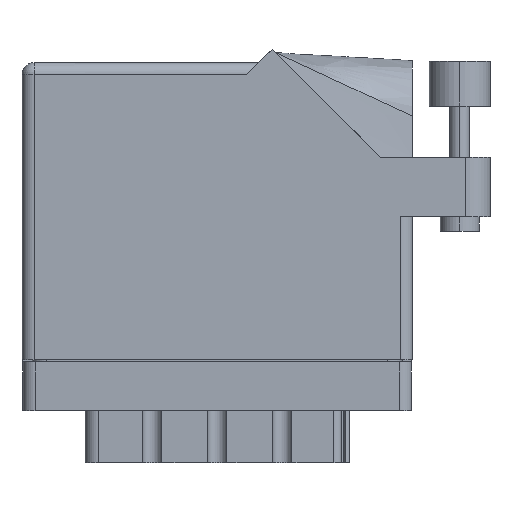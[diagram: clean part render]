
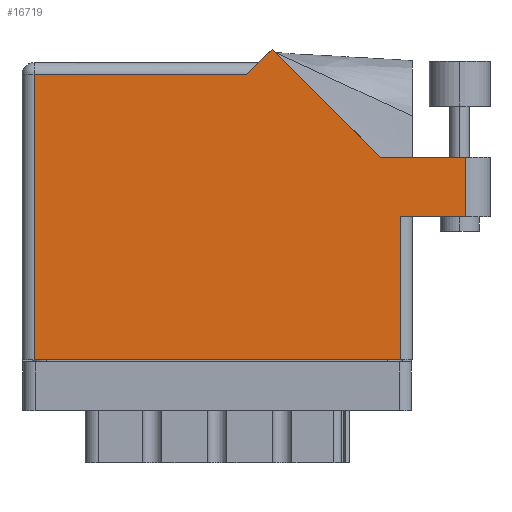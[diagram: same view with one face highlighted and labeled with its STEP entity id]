
A CAD part, front view. The second image highlights one B-rep face of the part: STEP entity #16719.
In plain terms, the highlighted face is planar.
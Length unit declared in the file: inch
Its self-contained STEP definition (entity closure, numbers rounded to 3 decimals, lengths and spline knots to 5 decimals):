
#139 = VERTEX_POINT ( 'NONE', #1897 ) ;
#693 = EDGE_CURVE ( 'NONE', #36157, #2123, #4992, .T. ) ;
#809 = CARTESIAN_POINT ( 'NONE',  ( 2.285, 1.044, 0. ) ) ;
#1897 = CARTESIAN_POINT ( 'NONE',  ( 1.948, 0., 0. ) ) ;
#2123 = VERTEX_POINT ( 'NONE', #23242 ) ;
#2434 = CARTESIAN_POINT ( 'NONE',  ( 1.155, 1.468, 0. ) ) ;
#3070 = VERTEX_POINT ( 'NONE', #40826 ) ;
#3728 = VERTEX_POINT ( 'NONE', #4222 ) ;
#4073 = VECTOR ( 'NONE', #17638, 39.37008 ) ;
#4222 = CARTESIAN_POINT ( 'NONE',  ( 0.062, 1.468, 0. ) ) ;
#4380 = CARTESIAN_POINT ( 'NONE',  ( 1.948, 0.737, 0. ) ) ;
#4992 = LINE ( 'NONE', #37120, #35378 ) ;
#5123 = VECTOR ( 'NONE', #17401, 39.37008 ) ;
#5252 = VERTEX_POINT ( 'NONE', #12595 ) ;
#5459 = EDGE_CURVE ( 'NONE', #139, #3070, #6660, .T. ) ;
#5875 = VERTEX_POINT ( 'NONE', #35113 ) ;
#5968 = DIRECTION ( 'NONE',  ( -1., 0., 0. ) ) ;
#6402 = DIRECTION ( 'NONE',  ( -1., 0., 0. ) ) ;
#6660 = LINE ( 'NONE', #4380, #40478 ) ;
#6796 = DIRECTION ( 'NONE',  ( 0., -1., 0. ) ) ;
#6895 = EDGE_CURVE ( 'NONE', #3070, #5252, #36879, .T. ) ;
#7743 = CARTESIAN_POINT ( 'NONE',  ( 2.01, 0.737, 0. ) ) ;
#8780 = LINE ( 'NONE', #33795, #28746 ) ;
#10447 = VECTOR ( 'NONE', #6796, 39.37008 ) ;
#10452 = CARTESIAN_POINT ( 'NONE',  ( 1.84442, 1.044, 0. ) ) ;
#10543 = EDGE_CURVE ( 'NONE', #2123, #13192, #39895, .T. ) ;
#10945 = DIRECTION ( 'NONE',  ( 1., 0., 0. ) ) ;
#11374 = CARTESIAN_POINT ( 'NONE',  ( 2.285, 1.044, 0. ) ) ;
#12034 = EDGE_CURVE ( 'NONE', #20595, #36157, #25389, .T. ) ;
#12595 = CARTESIAN_POINT ( 'NONE',  ( 2.285, 0.737, 0. ) ) ;
#13192 = VERTEX_POINT ( 'NONE', #2434 ) ;
#13407 = EDGE_LOOP ( 'NONE', ( #14334, #23855, #37479, #35496, #15533, #14873, #13484, #30137, #29084 ) ) ;
#13484 = ORIENTED_EDGE ( 'NONE', *, *, #17842, .T. ) ;
#13497 = VECTOR ( 'NONE', #10945, 39.37008 ) ;
#14334 = ORIENTED_EDGE ( 'NONE', *, *, #6895, .T. ) ;
#14409 = CARTESIAN_POINT ( 'NONE',  ( 1.217, 1.53, 0. ) ) ;
#14873 = ORIENTED_EDGE ( 'NONE', *, *, #29199, .T. ) ;
#15533 = ORIENTED_EDGE ( 'NONE', *, *, #10543, .T. ) ;
#15965 = LINE ( 'NONE', #25849, #10447 ) ;
#16445 = VECTOR ( 'NONE', #6402, 39.37008 ) ;
#16719 = ADVANCED_FACE ( 'NONE', ( #32249 ), #24894, .F. ) ;
#17401 = DIRECTION ( 'NONE',  ( 0., 1., 0. ) ) ;
#17638 = DIRECTION ( 'NONE',  ( -0.707, -0.707, 0. ) ) ;
#17842 = EDGE_CURVE ( 'NONE', #3728, #5875, #15965, .T. ) ;
#20595 = VERTEX_POINT ( 'NONE', #11374 ) ;
#23242 = CARTESIAN_POINT ( 'NONE',  ( 1.28771, 1.60071, 0. ) ) ;
#23855 = ORIENTED_EDGE ( 'NONE', *, *, #27648, .T. ) ;
#24351 = DIRECTION ( 'NONE',  ( -0.707, 0.707, 0. ) ) ;
#24894 = PLANE ( 'NONE',  #34003 ) ;
#25389 = LINE ( 'NONE', #25464, #16445 ) ;
#25464 = CARTESIAN_POINT ( 'NONE',  ( 2.41, 1.044, 0. ) ) ;
#25849 = CARTESIAN_POINT ( 'NONE',  ( 0.062, 0., 0. ) ) ;
#26364 = VECTOR ( 'NONE', #31469, 39.37008 ) ;
#27648 = EDGE_CURVE ( 'NONE', #5252, #20595, #32977, .T. ) ;
#28746 = VECTOR ( 'NONE', #37788, 39.37008 ) ;
#29084 = ORIENTED_EDGE ( 'NONE', *, *, #5459, .T. ) ;
#29199 = EDGE_CURVE ( 'NONE', #13192, #3728, #35820, .T. ) ;
#30137 = ORIENTED_EDGE ( 'NONE', *, *, #31754, .T. ) ;
#31206 = CARTESIAN_POINT ( 'NONE',  ( 0., 1.468, 0. ) ) ;
#31469 = DIRECTION ( 'NONE',  ( -1., 0., 0. ) ) ;
#31754 = EDGE_CURVE ( 'NONE', #5875, #139, #8780, .T. ) ;
#32249 = FACE_OUTER_BOUND ( 'NONE', #13407, .T. ) ;
#32775 = DIRECTION ( 'NONE',  ( 0., 1., 0. ) ) ;
#32977 = LINE ( 'NONE', #809, #5123 ) ;
#33795 = CARTESIAN_POINT ( 'NONE',  ( 0., 0., 0. ) ) ;
#34003 = AXIS2_PLACEMENT_3D ( 'NONE', #37796, #38223, #5968 ) ;
#35113 = CARTESIAN_POINT ( 'NONE',  ( 0.062, 0., 0. ) ) ;
#35378 = VECTOR ( 'NONE', #24351, 39.37008 ) ;
#35496 = ORIENTED_EDGE ( 'NONE', *, *, #693, .T. ) ;
#35820 = LINE ( 'NONE', #31206, #26364 ) ;
#36157 = VERTEX_POINT ( 'NONE', #10452 ) ;
#36879 = LINE ( 'NONE', #7743, #13497 ) ;
#37120 = CARTESIAN_POINT ( 'NONE',  ( 1.84442, 1.044, 0. ) ) ;
#37479 = ORIENTED_EDGE ( 'NONE', *, *, #12034, .T. ) ;
#37788 = DIRECTION ( 'NONE',  ( 1., 0., 0. ) ) ;
#37796 = CARTESIAN_POINT ( 'NONE',  ( 0., 1.53, 0. ) ) ;
#38223 = DIRECTION ( 'NONE',  ( 0., 0., -1. ) ) ;
#39895 = LINE ( 'NONE', #14409, #4073 ) ;
#40478 = VECTOR ( 'NONE', #32775, 39.37008 ) ;
#40826 = CARTESIAN_POINT ( 'NONE',  ( 1.948, 0.737, 0. ) ) ;
